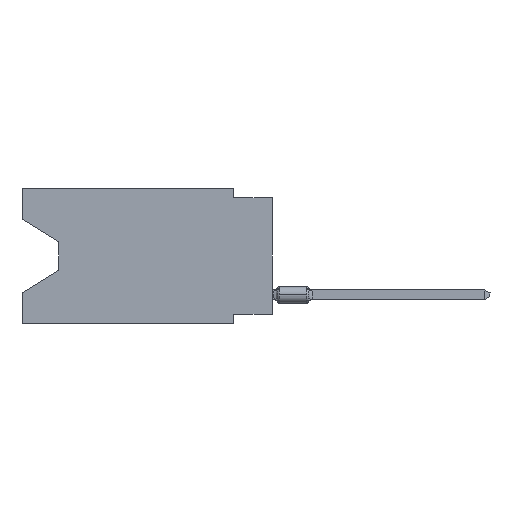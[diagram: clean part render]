
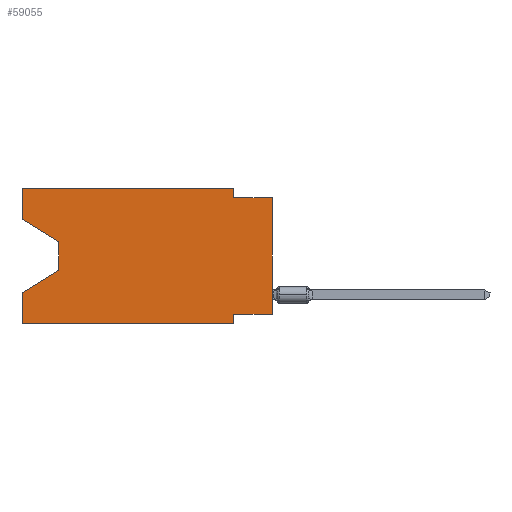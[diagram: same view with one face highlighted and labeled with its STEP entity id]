
A CAD part, left-side view. The second image highlights one B-rep face of the part: STEP entity #59055.
In plain terms, the highlighted planar face has unit normal (-1, 0, 0).
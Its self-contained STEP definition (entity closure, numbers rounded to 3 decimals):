
#5119 = VECTOR ( 'NONE', #81810, 1000. ) ;
#6447 = CARTESIAN_POINT ( 'NONE',  ( 0., 16.383, 0. ) ) ;
#7636 = VERTEX_POINT ( 'NONE', #39215 ) ;
#9562 = ORIENTED_EDGE ( 'NONE', *, *, #38905, .T. ) ;
#10639 = VERTEX_POINT ( 'NONE', #35058 ) ;
#11486 = EDGE_CURVE ( 'NONE', #39766, #11931, #73108, .T. ) ;
#11931 = VERTEX_POINT ( 'NONE', #40086 ) ;
#12254 = EDGE_CURVE ( 'NONE', #45934, #25312, #39538, .T. ) ;
#12831 = VECTOR ( 'NONE', #56823, 1000. ) ;
#13205 = VECTOR ( 'NONE', #43111, 1000. ) ;
#13495 = ORIENTED_EDGE ( 'NONE', *, *, #27189, .F. ) ;
#13563 = CARTESIAN_POINT ( 'NONE',  ( 0., 16.383, -8.89 ) ) ;
#14277 = ORIENTED_EDGE ( 'NONE', *, *, #55610, .T. ) ;
#14767 = DIRECTION ( 'NONE',  ( 0., 0., -1. ) ) ;
#15372 = LINE ( 'NONE', #42836, #69271 ) ;
#15666 = EDGE_CURVE ( 'NONE', #45934, #35278, #57506, .T. ) ;
#21219 = CARTESIAN_POINT ( 'NONE',  ( 0., 13.97, -3.505 ) ) ;
#21258 = DIRECTION ( 'NONE',  ( 0., 0., -1. ) ) ;
#23562 = DIRECTION ( 'NONE',  ( 0., 1., 0. ) ) ;
#23626 = LINE ( 'NONE', #44307, #34099 ) ;
#23914 = EDGE_LOOP ( 'NONE', ( #29460, #14277, #84534, #29528, #80822, #30206, #58329, #9562, #34730, #13495, #33813, #50449 ) ) ;
#24943 = DIRECTION ( 'NONE',  ( 0., -1., 0. ) ) ;
#25312 = VERTEX_POINT ( 'NONE', #83096 ) ;
#27189 = EDGE_CURVE ( 'NONE', #7636, #61633, #29170, .T. ) ;
#28935 = CARTESIAN_POINT ( 'NONE',  ( 0., 16.383, -2.038 ) ) ;
#29170 = LINE ( 'NONE', #57060, #13205 ) ;
#29359 = LINE ( 'NONE', #50505, #12831 ) ;
#29460 = ORIENTED_EDGE ( 'NONE', *, *, #15666, .T. ) ;
#29528 = ORIENTED_EDGE ( 'NONE', *, *, #78996, .F. ) ;
#30206 = ORIENTED_EDGE ( 'NONE', *, *, #78431, .F. ) ;
#30762 = CARTESIAN_POINT ( 'NONE',  ( 0., 0., -0.635 ) ) ;
#30771 = CARTESIAN_POINT ( 'NONE',  ( 0., 0., -8.255 ) ) ;
#31574 = VERTEX_POINT ( 'NONE', #79250 ) ;
#33813 = ORIENTED_EDGE ( 'NONE', *, *, #67706, .F. ) ;
#34099 = VECTOR ( 'NONE', #38900, 1000. ) ;
#34338 = FACE_OUTER_BOUND ( 'NONE', #23914, .T. ) ;
#34730 = ORIENTED_EDGE ( 'NONE', *, *, #38203, .F. ) ;
#35058 = CARTESIAN_POINT ( 'NONE',  ( 0., 16.383, -6.852 ) ) ;
#35278 = VERTEX_POINT ( 'NONE', #21219 ) ;
#37379 = VECTOR ( 'NONE', #24943, 1000. ) ;
#37415 = LINE ( 'NONE', #44608, #65793 ) ;
#38203 = EDGE_CURVE ( 'NONE', #61633, #80056, #29359, .T. ) ;
#38900 = DIRECTION ( 'NONE',  ( 0., 0., 1. ) ) ;
#38905 = EDGE_CURVE ( 'NONE', #80356, #80056, #46201, .T. ) ;
#39215 = CARTESIAN_POINT ( 'NONE',  ( 0., 2.54, 0. ) ) ;
#39538 = LINE ( 'NONE', #45854, #67457 ) ;
#39766 = VERTEX_POINT ( 'NONE', #13563 ) ;
#40086 = CARTESIAN_POINT ( 'NONE',  ( 0., 2.54, -8.89 ) ) ;
#41097 = DIRECTION ( 'NONE',  ( 1., 0., 0. ) ) ;
#41396 = VECTOR ( 'NONE', #23562, 1000. ) ;
#42836 = CARTESIAN_POINT ( 'NONE',  ( 0., 13.97, -3.505 ) ) ;
#43111 = DIRECTION ( 'NONE',  ( 0., 0., -1. ) ) ;
#43787 = VECTOR ( 'NONE', #48968, 1000. ) ;
#44307 = CARTESIAN_POINT ( 'NONE',  ( 0., 16.383, 0. ) ) ;
#44608 = CARTESIAN_POINT ( 'NONE',  ( 0., 13.97, -5.385 ) ) ;
#45854 = CARTESIAN_POINT ( 'NONE',  ( 0., 16.383, 0. ) ) ;
#45934 = VERTEX_POINT ( 'NONE', #28935 ) ;
#46201 = LINE ( 'NONE', #53858, #70342 ) ;
#48287 = PLANE ( 'NONE',  #69525 ) ;
#48968 = DIRECTION ( 'NONE',  ( 0., -0.855, -0.519 ) ) ;
#49607 = EDGE_CURVE ( 'NONE', #80356, #31574, #71297, .T. ) ;
#50449 = ORIENTED_EDGE ( 'NONE', *, *, #12254, .F. ) ;
#50505 = CARTESIAN_POINT ( 'NONE',  ( 0., 0., -0.635 ) ) ;
#51935 = CARTESIAN_POINT ( 'NONE',  ( 0., 13.97, -5.385 ) ) ;
#53412 = DIRECTION ( 'NONE',  ( 0., 0., 1. ) ) ;
#53858 = CARTESIAN_POINT ( 'NONE',  ( 0., 0., 0. ) ) ;
#55610 = EDGE_CURVE ( 'NONE', #35278, #71723, #15372, .T. ) ;
#56823 = DIRECTION ( 'NONE',  ( 0., -1., 0. ) ) ;
#57060 = CARTESIAN_POINT ( 'NONE',  ( 0., 2.54, 0. ) ) ;
#57506 = LINE ( 'NONE', #84988, #43787 ) ;
#58329 = ORIENTED_EDGE ( 'NONE', *, *, #49607, .F. ) ;
#59055 = ADVANCED_FACE ( 'NONE', ( #34338 ), #48287, .F. ) ;
#61633 = VERTEX_POINT ( 'NONE', #77825 ) ;
#64903 = DIRECTION ( 'NONE',  ( 0., 0.855, -0.519 ) ) ;
#65697 = DIRECTION ( 'NONE',  ( 0., 0., 1. ) ) ;
#65793 = VECTOR ( 'NONE', #64903, 1000. ) ;
#65906 = CARTESIAN_POINT ( 'NONE',  ( 0., 16.383, -8.89 ) ) ;
#67457 = VECTOR ( 'NONE', #65697, 1000. ) ;
#67706 = EDGE_CURVE ( 'NONE', #25312, #7636, #80930, .T. ) ;
#68568 = DIRECTION ( 'NONE',  ( 0., 0., -1. ) ) ;
#69260 = LINE ( 'NONE', #69695, #84382 ) ;
#69271 = VECTOR ( 'NONE', #21258, 1000. ) ;
#69525 = AXIS2_PLACEMENT_3D ( 'NONE', #6447, #41097, #68568 ) ;
#69695 = CARTESIAN_POINT ( 'NONE',  ( 0., 2.54, -8.89 ) ) ;
#69924 = EDGE_CURVE ( 'NONE', #71723, #10639, #37415, .T. ) ;
#70342 = VECTOR ( 'NONE', #53412, 1000. ) ;
#71297 = LINE ( 'NONE', #30771, #41396 ) ;
#71723 = VERTEX_POINT ( 'NONE', #51935 ) ;
#73108 = LINE ( 'NONE', #65906, #37379 ) ;
#74164 = CARTESIAN_POINT ( 'NONE',  ( 0., 16.383, 0. ) ) ;
#77825 = CARTESIAN_POINT ( 'NONE',  ( 0., 2.54, -0.635 ) ) ;
#78431 = EDGE_CURVE ( 'NONE', #31574, #11931, #69260, .T. ) ;
#78996 = EDGE_CURVE ( 'NONE', #39766, #10639, #23626, .T. ) ;
#79250 = CARTESIAN_POINT ( 'NONE',  ( 0., 2.54, -8.255 ) ) ;
#80056 = VERTEX_POINT ( 'NONE', #30762 ) ;
#80356 = VERTEX_POINT ( 'NONE', #84676 ) ;
#80822 = ORIENTED_EDGE ( 'NONE', *, *, #11486, .T. ) ;
#80930 = LINE ( 'NONE', #74164, #5119 ) ;
#81810 = DIRECTION ( 'NONE',  ( 0., -1., 0. ) ) ;
#83096 = CARTESIAN_POINT ( 'NONE',  ( 0., 16.383, 0. ) ) ;
#84382 = VECTOR ( 'NONE', #14767, 1000. ) ;
#84534 = ORIENTED_EDGE ( 'NONE', *, *, #69924, .T. ) ;
#84676 = CARTESIAN_POINT ( 'NONE',  ( 0., 0., -8.255 ) ) ;
#84988 = CARTESIAN_POINT ( 'NONE',  ( 0., 16.383, -2.038 ) ) ;
